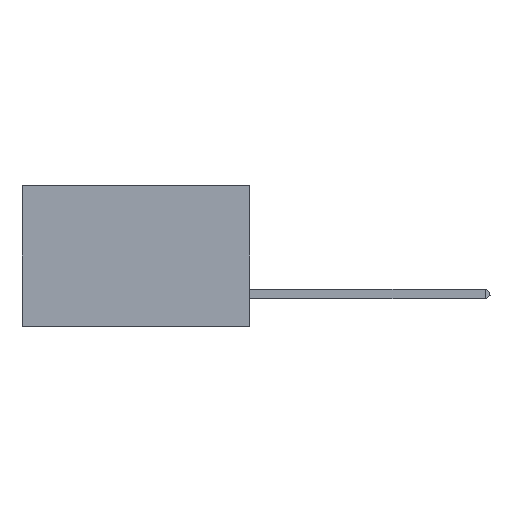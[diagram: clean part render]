
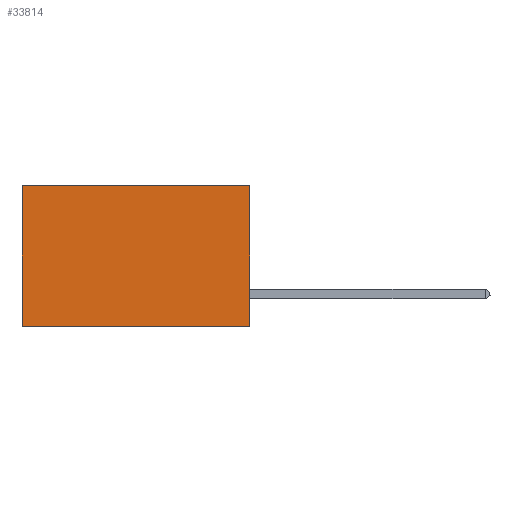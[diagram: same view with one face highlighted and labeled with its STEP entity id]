
A CAD part, left-side view. The second image highlights one B-rep face of the part: STEP entity #33814.
In plain terms, the highlighted planar face has unit normal (-1, 0, 0).
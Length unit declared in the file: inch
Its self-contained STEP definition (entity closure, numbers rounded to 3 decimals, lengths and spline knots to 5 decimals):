
#1322 = LINE ( 'NONE', #34215, #25169 ) ;
#1501 = CARTESIAN_POINT ( 'NONE',  ( 0.2875, 0., 0. ) ) ;
#2066 = PLANE ( 'NONE',  #43115 ) ;
#2154 = CARTESIAN_POINT ( 'NONE',  ( 0.2875, 0.6, -0.37 ) ) ;
#4788 = CARTESIAN_POINT ( 'NONE',  ( 0.2875, 0., -0.37 ) ) ;
#4836 = ORIENTED_EDGE ( 'NONE', *, *, #6653, .T. ) ;
#4973 = EDGE_LOOP ( 'NONE', ( #4836, #10468, #37801, #22225 ) ) ;
#4991 = EDGE_CURVE ( 'NONE', #15748, #39860, #10846, .T. ) ;
#5835 = CARTESIAN_POINT ( 'NONE',  ( 0.2875, 0., 0. ) ) ;
#6307 = DIRECTION ( 'NONE',  ( 0., 0., -1. ) ) ;
#6653 = EDGE_CURVE ( 'NONE', #39860, #31539, #1322, .T. ) ;
#8466 = DIRECTION ( 'NONE',  ( 0., 0., -1. ) ) ;
#10021 = LINE ( 'NONE', #4788, #37971 ) ;
#10468 = ORIENTED_EDGE ( 'NONE', *, *, #43007, .F. ) ;
#10846 = LINE ( 'NONE', #1501, #28224 ) ;
#11442 = LINE ( 'NONE', #18885, #31106 ) ;
#15748 = VERTEX_POINT ( 'NONE', #35425 ) ;
#18885 = CARTESIAN_POINT ( 'NONE',  ( 0.2875, 0., 0. ) ) ;
#20059 = EDGE_CURVE ( 'NONE', #15748, #28145, #11442, .T. ) ;
#21155 = FACE_OUTER_BOUND ( 'NONE', #4973, .T. ) ;
#22130 = DIRECTION ( 'NONE',  ( 0., 0., -1. ) ) ;
#22225 = ORIENTED_EDGE ( 'NONE', *, *, #4991, .T. ) ;
#24939 = DIRECTION ( 'NONE',  ( 1., 0., 0. ) ) ;
#25169 = VECTOR ( 'NONE', #8466, 39.37008 ) ;
#28145 = VERTEX_POINT ( 'NONE', #37913 ) ;
#28224 = VECTOR ( 'NONE', #38881, 39.37008 ) ;
#31106 = VECTOR ( 'NONE', #22130, 39.37008 ) ;
#31539 = VERTEX_POINT ( 'NONE', #2154 ) ;
#33814 = ADVANCED_FACE ( 'NONE', ( #21155 ), #2066, .F. ) ;
#34215 = CARTESIAN_POINT ( 'NONE',  ( 0.2875, 0.6, 0. ) ) ;
#34419 = DIRECTION ( 'NONE',  ( 0., 1., 0. ) ) ;
#35425 = CARTESIAN_POINT ( 'NONE',  ( 0.2875, 0., 0. ) ) ;
#37801 = ORIENTED_EDGE ( 'NONE', *, *, #20059, .F. ) ;
#37913 = CARTESIAN_POINT ( 'NONE',  ( 0.2875, 0., -0.37 ) ) ;
#37971 = VECTOR ( 'NONE', #34419, 39.37008 ) ;
#38881 = DIRECTION ( 'NONE',  ( 0., 1., 0. ) ) ;
#39860 = VERTEX_POINT ( 'NONE', #42472 ) ;
#42472 = CARTESIAN_POINT ( 'NONE',  ( 0.2875, 0.6, 0. ) ) ;
#43007 = EDGE_CURVE ( 'NONE', #28145, #31539, #10021, .T. ) ;
#43115 = AXIS2_PLACEMENT_3D ( 'NONE', #5835, #24939, #6307 ) ;
